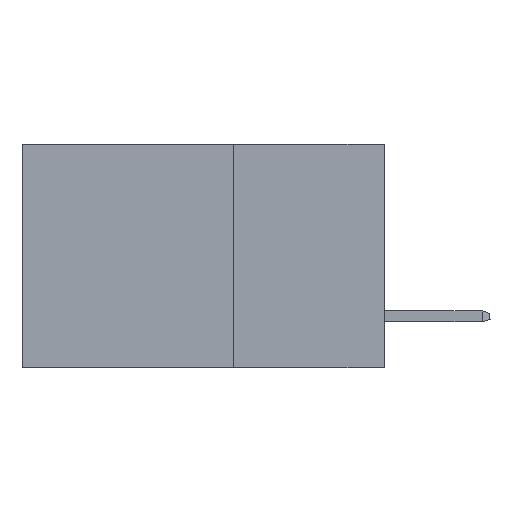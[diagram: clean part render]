
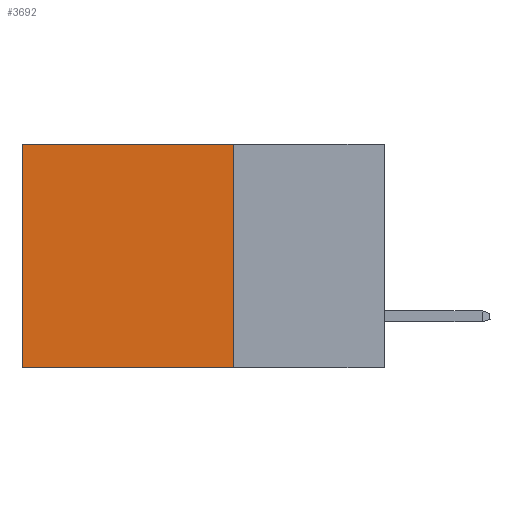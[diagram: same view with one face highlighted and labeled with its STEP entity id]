
A CAD part, left-side view. The second image highlights one B-rep face of the part: STEP entity #3692.
In plain terms, the highlighted planar face has unit normal (-1, 0, 0).
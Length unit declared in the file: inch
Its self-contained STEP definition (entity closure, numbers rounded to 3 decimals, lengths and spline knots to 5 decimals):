
#156 = VECTOR ( 'NONE', #1771, 39.37008 ) ;
#472 = ORIENTED_EDGE ( 'NONE', *, *, #2994, .T. ) ;
#526 = CARTESIAN_POINT ( 'NONE',  ( 0.298, 0.25, 0. ) ) ;
#1005 = FACE_OUTER_BOUND ( 'NONE', #6038, .T. ) ;
#1189 = CARTESIAN_POINT ( 'NONE',  ( 0.298, 0.6, 0. ) ) ;
#1262 = DIRECTION ( 'NONE',  ( 1., 0., 0. ) ) ;
#1359 = EDGE_CURVE ( 'NONE', #5546, #2838, #5523, .T. ) ;
#1396 = DIRECTION ( 'NONE',  ( 0., 0., -1. ) ) ;
#1498 = VECTOR ( 'NONE', #5530, 39.37008 ) ;
#1552 = CARTESIAN_POINT ( 'NONE',  ( 0.298, 0.25, 0. ) ) ;
#1771 = DIRECTION ( 'NONE',  ( 0., 1., 0. ) ) ;
#2359 = CARTESIAN_POINT ( 'NONE',  ( 0.298, 0.25, 0. ) ) ;
#2704 = CARTESIAN_POINT ( 'NONE',  ( 0.298, 0.25, 0. ) ) ;
#2838 = VERTEX_POINT ( 'NONE', #4366 ) ;
#2976 = ORIENTED_EDGE ( 'NONE', *, *, #7982, .F. ) ;
#2994 = EDGE_CURVE ( 'NONE', #4962, #2838, #9810, .T. ) ;
#3692 = ADVANCED_FACE ( 'NONE', ( #1005 ), #5082, .F. ) ;
#4268 = DIRECTION ( 'NONE',  ( 0., 1., 0. ) ) ;
#4366 = CARTESIAN_POINT ( 'NONE',  ( 0.298, 0.6, -0.37 ) ) ;
#4867 = AXIS2_PLACEMENT_3D ( 'NONE', #526, #1262, #1396 ) ;
#4962 = VERTEX_POINT ( 'NONE', #1189 ) ;
#5082 = PLANE ( 'NONE',  #4867 ) ;
#5523 = LINE ( 'NONE', #6377, #156 ) ;
#5530 = DIRECTION ( 'NONE',  ( 0., 0., -1. ) ) ;
#5546 = VERTEX_POINT ( 'NONE', #9823 ) ;
#5864 = LINE ( 'NONE', #2359, #6082 ) ;
#6038 = EDGE_LOOP ( 'NONE', ( #472, #6170, #2976, #6633 ) ) ;
#6082 = VECTOR ( 'NONE', #8409, 39.37008 ) ;
#6170 = ORIENTED_EDGE ( 'NONE', *, *, #1359, .F. ) ;
#6361 = CARTESIAN_POINT ( 'NONE',  ( 0.298, 0.6, 0. ) ) ;
#6377 = CARTESIAN_POINT ( 'NONE',  ( 0.298, 0.25, -0.37 ) ) ;
#6633 = ORIENTED_EDGE ( 'NONE', *, *, #9728, .T. ) ;
#7573 = LINE ( 'NONE', #2704, #9441 ) ;
#7982 = EDGE_CURVE ( 'NONE', #9800, #5546, #5864, .T. ) ;
#8409 = DIRECTION ( 'NONE',  ( 0., 0., -1. ) ) ;
#9441 = VECTOR ( 'NONE', #4268, 39.37008 ) ;
#9728 = EDGE_CURVE ( 'NONE', #9800, #4962, #7573, .T. ) ;
#9800 = VERTEX_POINT ( 'NONE', #1552 ) ;
#9810 = LINE ( 'NONE', #6361, #1498 ) ;
#9823 = CARTESIAN_POINT ( 'NONE',  ( 0.298, 0.25, -0.37 ) ) ;
